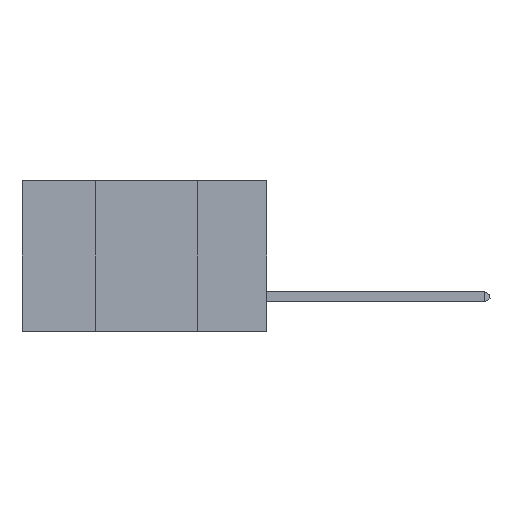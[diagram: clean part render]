
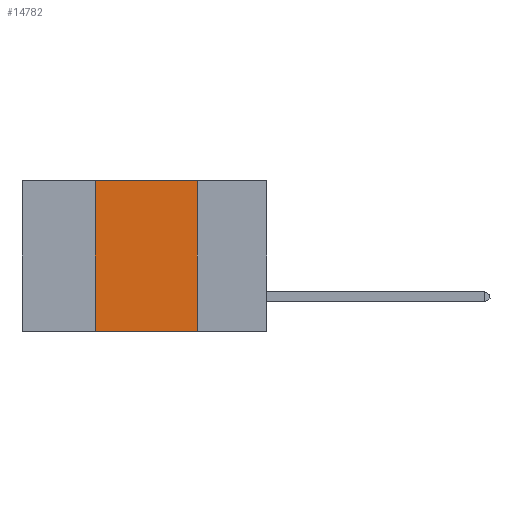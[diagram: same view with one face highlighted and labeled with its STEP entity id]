
A CAD part, left-side view. The second image highlights one B-rep face of the part: STEP entity #14782.
In plain terms, the highlighted planar face has unit normal (-1, 0, 0).
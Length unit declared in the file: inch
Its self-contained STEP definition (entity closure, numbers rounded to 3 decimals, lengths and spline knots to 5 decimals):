
#2553 = DIRECTION ( 'NONE',  ( 1., 0., 0. ) ) ;
#3372 = CARTESIAN_POINT ( 'NONE',  ( 0., 0.6, 0. ) ) ;
#4099 = CARTESIAN_POINT ( 'NONE',  ( 0., 0.17, -0.37 ) ) ;
#4549 = LINE ( 'NONE', #23153, #9788 ) ;
#4867 = AXIS2_PLACEMENT_3D ( 'NONE', #14355, #2553, #16270 ) ;
#5493 = CARTESIAN_POINT ( 'NONE',  ( 0., 0.6, -0.37 ) ) ;
#6205 = VECTOR ( 'NONE', #11456, 39.37008 ) ;
#8366 = EDGE_CURVE ( 'NONE', #8799, #19665, #16048, .T. ) ;
#8799 = VERTEX_POINT ( 'NONE', #10749 ) ;
#8860 = EDGE_CURVE ( 'NONE', #8799, #23416, #21003, .T. ) ;
#9788 = VECTOR ( 'NONE', #19414, 39.37008 ) ;
#10373 = PLANE ( 'NONE',  #4867 ) ;
#10749 = CARTESIAN_POINT ( 'NONE',  ( 0., 0.42, -0.37 ) ) ;
#10973 = ORIENTED_EDGE ( 'NONE', *, *, #13192, .F. ) ;
#11456 = DIRECTION ( 'NONE',  ( 0., -1., 0. ) ) ;
#11524 = VERTEX_POINT ( 'NONE', #16568 ) ;
#12806 = FACE_OUTER_BOUND ( 'NONE', #20906, .T. ) ;
#13192 = EDGE_CURVE ( 'NONE', #11524, #19665, #4549, .T. ) ;
#14240 = VECTOR ( 'NONE', #17151, 39.37008 ) ;
#14355 = CARTESIAN_POINT ( 'NONE',  ( 0., 0.6, 0. ) ) ;
#14370 = ORIENTED_EDGE ( 'NONE', *, *, #22047, .F. ) ;
#14782 = ADVANCED_FACE ( 'NONE', ( #12806 ), #10373, .F. ) ;
#15423 = VECTOR ( 'NONE', #24140, 39.37008 ) ;
#16048 = LINE ( 'NONE', #5493, #6205 ) ;
#16270 = DIRECTION ( 'NONE',  ( 0., 0., -1. ) ) ;
#16538 = CARTESIAN_POINT ( 'NONE',  ( 0., 0.42, 0. ) ) ;
#16568 = CARTESIAN_POINT ( 'NONE',  ( 0., 0.17, 0. ) ) ;
#17011 = ORIENTED_EDGE ( 'NONE', *, *, #8860, .F. ) ;
#17151 = DIRECTION ( 'NONE',  ( 0., -1., 0. ) ) ;
#18106 = ORIENTED_EDGE ( 'NONE', *, *, #8366, .T. ) ;
#19239 = LINE ( 'NONE', #3372, #14240 ) ;
#19414 = DIRECTION ( 'NONE',  ( 0., 0., -1. ) ) ;
#19665 = VERTEX_POINT ( 'NONE', #4099 ) ;
#20906 = EDGE_LOOP ( 'NONE', ( #10973, #14370, #17011, #18106 ) ) ;
#21003 = LINE ( 'NONE', #22330, #15423 ) ;
#22047 = EDGE_CURVE ( 'NONE', #23416, #11524, #19239, .T. ) ;
#22330 = CARTESIAN_POINT ( 'NONE',  ( 0., 0.42, 0. ) ) ;
#23153 = CARTESIAN_POINT ( 'NONE',  ( 0., 0.17, 0. ) ) ;
#23416 = VERTEX_POINT ( 'NONE', #16538 ) ;
#24140 = DIRECTION ( 'NONE',  ( 0., 0., 1. ) ) ;
